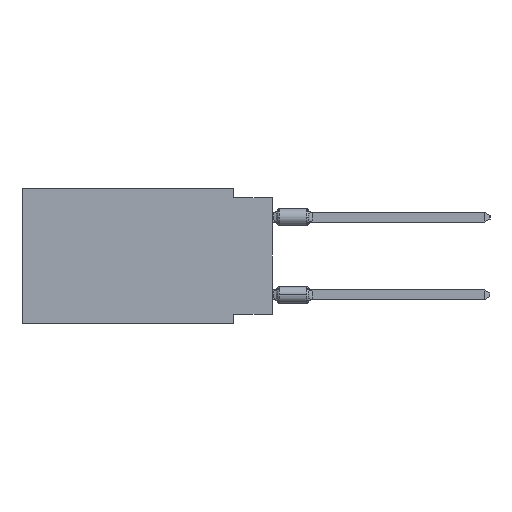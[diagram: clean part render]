
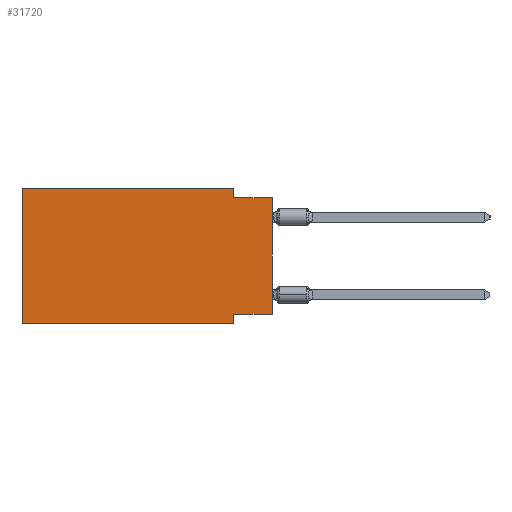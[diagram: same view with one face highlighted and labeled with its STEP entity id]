
A CAD part, left-side view. The second image highlights one B-rep face of the part: STEP entity #31720.
In plain terms, the highlighted planar face has unit normal (-1, 0, 0).
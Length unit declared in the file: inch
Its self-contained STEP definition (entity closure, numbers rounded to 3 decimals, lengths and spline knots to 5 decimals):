
#53 = PLANE ( 'NONE',  #48895 ) ;
#569 = VECTOR ( 'NONE', #59087, 39.37008 ) ;
#570 = CARTESIAN_POINT ( 'NONE',  ( 0., 0.645, -0.35 ) ) ;
#1051 = VERTEX_POINT ( 'NONE', #570 ) ;
#1109 = EDGE_CURVE ( 'NONE', #44615, #27906, #24317, .T. ) ;
#1465 = CARTESIAN_POINT ( 'NONE',  ( 0., 0.1, 0. ) ) ;
#2128 = CARTESIAN_POINT ( 'NONE',  ( 0., 0.1, -0.025 ) ) ;
#2353 = CARTESIAN_POINT ( 'NONE',  ( 0., 0., 0. ) ) ;
#2435 = LINE ( 'NONE', #39732, #10318 ) ;
#4178 = CARTESIAN_POINT ( 'NONE',  ( 0., 0.1, -0.35 ) ) ;
#4276 = LINE ( 'NONE', #54830, #25093 ) ;
#4668 = ORIENTED_EDGE ( 'NONE', *, *, #13913, .F. ) ;
#4998 = VECTOR ( 'NONE', #20699, 39.37008 ) ;
#6421 = VECTOR ( 'NONE', #55429, 39.37008 ) ;
#8513 = CARTESIAN_POINT ( 'NONE',  ( 0., 0., -0.325 ) ) ;
#8673 = EDGE_CURVE ( 'NONE', #30483, #20121, #11991, .T. ) ;
#9130 = VECTOR ( 'NONE', #11394, 39.37008 ) ;
#9247 = CARTESIAN_POINT ( 'NONE',  ( 0., 0., -0.025 ) ) ;
#10318 = VECTOR ( 'NONE', #34639, 39.37008 ) ;
#11394 = DIRECTION ( 'NONE',  ( 0., 0., -1. ) ) ;
#11991 = LINE ( 'NONE', #16792, #9130 ) ;
#12265 = EDGE_CURVE ( 'NONE', #1051, #14587, #2435, .T. ) ;
#13070 = ORIENTED_EDGE ( 'NONE', *, *, #1109, .F. ) ;
#13900 = LINE ( 'NONE', #8513, #6421 ) ;
#13913 = EDGE_CURVE ( 'NONE', #14587, #44615, #32685, .T. ) ;
#14587 = VERTEX_POINT ( 'NONE', #44012 ) ;
#16792 = CARTESIAN_POINT ( 'NONE',  ( 0., 0.1, -0.35 ) ) ;
#18176 = VERTEX_POINT ( 'NONE', #9247 ) ;
#18377 = EDGE_LOOP ( 'NONE', ( #28492, #47979, #13070, #4668, #18959, #35566, #40408, #54529 ) ) ;
#18501 = EDGE_CURVE ( 'NONE', #26535, #30483, #13900, .T. ) ;
#18959 = ORIENTED_EDGE ( 'NONE', *, *, #12265, .F. ) ;
#19629 = VECTOR ( 'NONE', #23063, 39.37008 ) ;
#20121 = VERTEX_POINT ( 'NONE', #4178 ) ;
#20699 = DIRECTION ( 'NONE',  ( 0., 0., 1. ) ) ;
#22400 = CARTESIAN_POINT ( 'NONE',  ( 0., 0.645, -0.35 ) ) ;
#22626 = DIRECTION ( 'NONE',  ( 0., -1., 0. ) ) ;
#23063 = DIRECTION ( 'NONE',  ( 0., -1., 0. ) ) ;
#24317 = LINE ( 'NONE', #1465, #49248 ) ;
#25093 = VECTOR ( 'NONE', #22626, 39.37008 ) ;
#26535 = VERTEX_POINT ( 'NONE', #27060 ) ;
#26875 = EDGE_CURVE ( 'NONE', #26535, #18176, #48071, .T. ) ;
#27060 = CARTESIAN_POINT ( 'NONE',  ( 0., 0., -0.325 ) ) ;
#27906 = VERTEX_POINT ( 'NONE', #2128 ) ;
#28109 = LINE ( 'NONE', #22400, #569 ) ;
#28492 = ORIENTED_EDGE ( 'NONE', *, *, #26875, .T. ) ;
#28737 = CARTESIAN_POINT ( 'NONE',  ( 0., 0.1, -0.325 ) ) ;
#30483 = VERTEX_POINT ( 'NONE', #28737 ) ;
#31720 = ADVANCED_FACE ( 'NONE', ( #41528 ), #53, .F. ) ;
#32685 = LINE ( 'NONE', #45924, #19629 ) ;
#34639 = DIRECTION ( 'NONE',  ( 0., 0., 1. ) ) ;
#35566 = ORIENTED_EDGE ( 'NONE', *, *, #53921, .T. ) ;
#39028 = DIRECTION ( 'NONE',  ( 0., 0., -1. ) ) ;
#39732 = CARTESIAN_POINT ( 'NONE',  ( 0., 0.645, 0. ) ) ;
#40408 = ORIENTED_EDGE ( 'NONE', *, *, #8673, .F. ) ;
#41528 = FACE_OUTER_BOUND ( 'NONE', #18377, .T. ) ;
#44012 = CARTESIAN_POINT ( 'NONE',  ( 0., 0.645, 0. ) ) ;
#44615 = VERTEX_POINT ( 'NONE', #50673 ) ;
#45924 = CARTESIAN_POINT ( 'NONE',  ( 0., 0.645, 0. ) ) ;
#47871 = EDGE_CURVE ( 'NONE', #27906, #18176, #4276, .T. ) ;
#47979 = ORIENTED_EDGE ( 'NONE', *, *, #47871, .F. ) ;
#48071 = LINE ( 'NONE', #2353, #4998 ) ;
#48895 = AXIS2_PLACEMENT_3D ( 'NONE', #55071, #55979, #50860 ) ;
#49248 = VECTOR ( 'NONE', #39028, 39.37008 ) ;
#50673 = CARTESIAN_POINT ( 'NONE',  ( 0., 0.1, 0. ) ) ;
#50860 = DIRECTION ( 'NONE',  ( 0., 0., -1. ) ) ;
#53921 = EDGE_CURVE ( 'NONE', #1051, #20121, #28109, .T. ) ;
#54529 = ORIENTED_EDGE ( 'NONE', *, *, #18501, .F. ) ;
#54830 = CARTESIAN_POINT ( 'NONE',  ( 0., 0., -0.025 ) ) ;
#55071 = CARTESIAN_POINT ( 'NONE',  ( 0., 0.645, 0. ) ) ;
#55429 = DIRECTION ( 'NONE',  ( 0., 1., 0. ) ) ;
#55979 = DIRECTION ( 'NONE',  ( 1., 0., 0. ) ) ;
#59087 = DIRECTION ( 'NONE',  ( 0., -1., 0. ) ) ;
